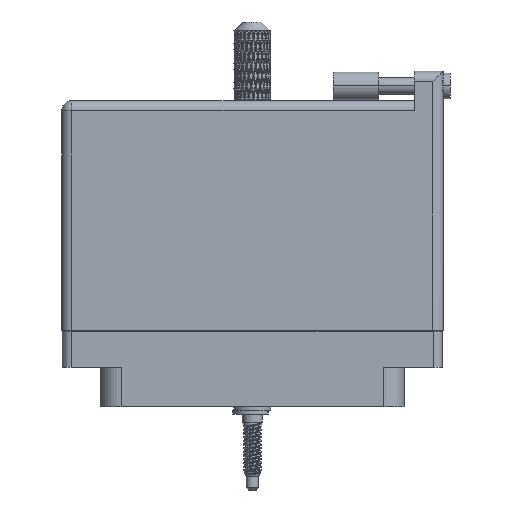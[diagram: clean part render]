
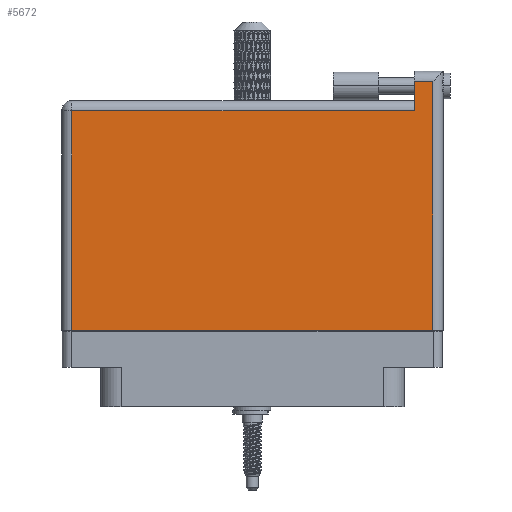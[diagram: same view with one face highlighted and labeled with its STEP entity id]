
A CAD part, front view. The second image highlights one B-rep face of the part: STEP entity #5672.
In plain terms, the highlighted face is planar.
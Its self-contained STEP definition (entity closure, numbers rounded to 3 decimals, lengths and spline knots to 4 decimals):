
#1015 = ORIENTED_EDGE ( 'NONE', *, *, #62102, .T. ) ;
#1075 = DIRECTION ( 'NONE',  ( 0., 1., 0. ) ) ;
#1140 = EDGE_CURVE ( 'NONE', #13617, #102867, #83690, .T. ) ;
#5169 = LINE ( 'NONE', #95553, #115736 ) ;
#5672 = ADVANCED_FACE ( 'NONE', ( #81680 ), #28145, .F. ) ;
#6012 = VECTOR ( 'NONE', #8605, 39.3701 ) ;
#8605 = DIRECTION ( 'NONE',  ( -1., 0., 0. ) ) ;
#8814 = CARTESIAN_POINT ( 'NONE',  ( 1.23, 1.666, 0.4495 ) ) ;
#10682 = AXIS2_PLACEMENT_3D ( 'NONE', #36508, #72750, #99497 ) ;
#13617 = VERTEX_POINT ( 'NONE', #77202 ) ;
#15321 = EDGE_CURVE ( 'NONE', #81512, #13617, #64995, .T. ) ;
#19858 = VECTOR ( 'NONE', #93725, 39.3701 ) ;
#21436 = VECTOR ( 'NONE', #23093, 39.3701 ) ;
#23093 = DIRECTION ( 'NONE',  ( -1., 0., 0. ) ) ;
#23938 = EDGE_LOOP ( 'NONE', ( #104936, #35466, #97090, #1015, #58322, #48653 ) ) ;
#26203 = CARTESIAN_POINT ( 'NONE',  ( 1.103, 1.596, 0.4495 ) ) ;
#28145 = PLANE ( 'NONE',  #10682 ) ;
#35466 = ORIENTED_EDGE ( 'NONE', *, *, #1140, .T. ) ;
#36508 = CARTESIAN_POINT ( 'NONE',  ( -1.3, 1.466, 0.4495 ) ) ;
#41677 = EDGE_CURVE ( 'NONE', #102867, #52119, #62749, .T. ) ;
#47463 = CARTESIAN_POINT ( 'NONE',  ( 1.23, 1.596, 0.4495 ) ) ;
#48403 = VERTEX_POINT ( 'NONE', #73706 ) ;
#48653 = ORIENTED_EDGE ( 'NONE', *, *, #110063, .T. ) ;
#52119 = VERTEX_POINT ( 'NONE', #26203 ) ;
#52428 = EDGE_CURVE ( 'NONE', #98857, #48403, #98409, .T. ) ;
#54429 = CARTESIAN_POINT ( 'NONE',  ( -1.3, 1.396, 0.4495 ) ) ;
#58322 = ORIENTED_EDGE ( 'NONE', *, *, #52428, .T. ) ;
#59134 = CARTESIAN_POINT ( 'NONE',  ( -1.23, -0.1, 0.4495 ) ) ;
#62102 = EDGE_CURVE ( 'NONE', #52119, #98857, #5169, .T. ) ;
#62749 = LINE ( 'NONE', #98969, #6012 ) ;
#64995 = LINE ( 'NONE', #94081, #116285 ) ;
#66964 = LINE ( 'NONE', #85970, #19858 ) ;
#72750 = DIRECTION ( 'NONE',  ( 0., 0., -1. ) ) ;
#73706 = CARTESIAN_POINT ( 'NONE',  ( -1.23, 1.396, 0.4495 ) ) ;
#75409 = DIRECTION ( 'NONE',  ( 0., -1., 0. ) ) ;
#77202 = CARTESIAN_POINT ( 'NONE',  ( 1.23, -0.1, 0.4495 ) ) ;
#81512 = VERTEX_POINT ( 'NONE', #59134 ) ;
#81680 = FACE_OUTER_BOUND ( 'NONE', #23938, .T. ) ;
#83690 = LINE ( 'NONE', #8814, #96718 ) ;
#84580 = DIRECTION ( 'NONE',  ( 1., 0., 0. ) ) ;
#85970 = CARTESIAN_POINT ( 'NONE',  ( -1.23, -0.1, 0.4495 ) ) ;
#93725 = DIRECTION ( 'NONE',  ( 0., -1., 0. ) ) ;
#94081 = CARTESIAN_POINT ( 'NONE',  ( -1.3, -0.1, 0.4495 ) ) ;
#95553 = CARTESIAN_POINT ( 'NONE',  ( 1.103, 1.666, 0.4495 ) ) ;
#96718 = VECTOR ( 'NONE', #1075, 39.3701 ) ;
#97090 = ORIENTED_EDGE ( 'NONE', *, *, #41677, .T. ) ;
#98409 = LINE ( 'NONE', #54429, #21436 ) ;
#98857 = VERTEX_POINT ( 'NONE', #103190 ) ;
#98969 = CARTESIAN_POINT ( 'NONE',  ( -1.3, 1.596, 0.4495 ) ) ;
#99497 = DIRECTION ( 'NONE',  ( -1., 0., 0. ) ) ;
#102867 = VERTEX_POINT ( 'NONE', #47463 ) ;
#103190 = CARTESIAN_POINT ( 'NONE',  ( 1.103, 1.396, 0.4495 ) ) ;
#104936 = ORIENTED_EDGE ( 'NONE', *, *, #15321, .T. ) ;
#110063 = EDGE_CURVE ( 'NONE', #48403, #81512, #66964, .T. ) ;
#115736 = VECTOR ( 'NONE', #75409, 39.3701 ) ;
#116285 = VECTOR ( 'NONE', #84580, 39.3701 ) ;
